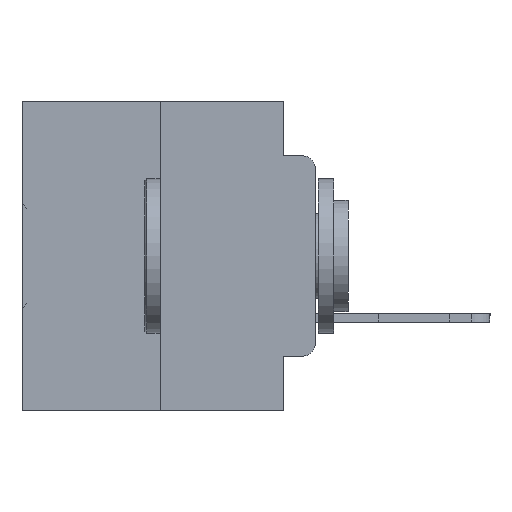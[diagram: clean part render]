
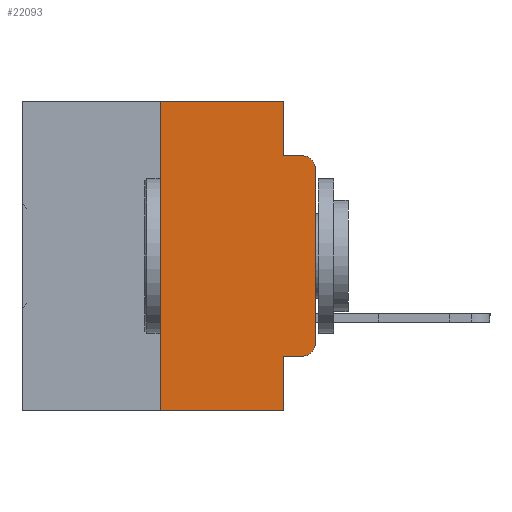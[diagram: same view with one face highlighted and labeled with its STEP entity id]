
A CAD part, left-side view. The second image highlights one B-rep face of the part: STEP entity #22093.
In plain terms, the highlighted planar face has unit normal (-1, 0, 0).
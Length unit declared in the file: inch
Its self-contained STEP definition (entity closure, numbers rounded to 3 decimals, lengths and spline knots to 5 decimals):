
#574 = DIRECTION ( 'NONE',  ( 0., -1., 0. ) ) ;
#651 = ORIENTED_EDGE ( 'NONE', *, *, #31635, .T. ) ;
#1986 = VERTEX_POINT ( 'NONE', #10382 ) ;
#2299 = LINE ( 'NONE', #29504, #22813 ) ;
#2353 = EDGE_CURVE ( 'NONE', #3374, #7126, #15050, .T. ) ;
#3009 = LINE ( 'NONE', #32769, #9323 ) ;
#3374 = VERTEX_POINT ( 'NONE', #23707 ) ;
#3595 = ORIENTED_EDGE ( 'NONE', *, *, #14703, .F. ) ;
#3640 = VERTEX_POINT ( 'NONE', #32210 ) ;
#3827 = VECTOR ( 'NONE', #5466, 39.37008 ) ;
#4020 = CARTESIAN_POINT ( 'NONE',  ( 0., 0.051, -0.4115 ) ) ;
#4184 = VERTEX_POINT ( 'NONE', #4714 ) ;
#4243 = DIRECTION ( 'NONE',  ( 0., 0., 1. ) ) ;
#4461 = PLANE ( 'NONE',  #11109 ) ;
#4573 = CARTESIAN_POINT ( 'NONE',  ( 0., 0.25, 0. ) ) ;
#4714 = CARTESIAN_POINT ( 'NONE',  ( 0., 0.02, -0.4115 ) ) ;
#4832 = EDGE_LOOP ( 'NONE', ( #13636, #28658, #15307, #29481, #3595, #25750, #12390, #14065, #28260, #651 ) ) ;
#5072 = CIRCLE ( 'NONE', #5090, 0.02 ) ;
#5090 = AXIS2_PLACEMENT_3D ( 'NONE', #6745, #25409, #9458 ) ;
#5247 = AXIS2_PLACEMENT_3D ( 'NONE', #12207, #30842, #14886 ) ;
#5418 = CARTESIAN_POINT ( 'NONE',  ( 0., 0.051, -0.5 ) ) ;
#5466 = DIRECTION ( 'NONE',  ( 0., -1., 0. ) ) ;
#5937 = DIRECTION ( 'NONE',  ( 0., 0., -1. ) ) ;
#5942 = CARTESIAN_POINT ( 'NONE',  ( 0., 0.051, 0. ) ) ;
#6423 = EDGE_CURVE ( 'NONE', #7899, #7126, #32448, .T. ) ;
#6745 = CARTESIAN_POINT ( 'NONE',  ( 0., 0.02, -0.1085 ) ) ;
#7126 = VERTEX_POINT ( 'NONE', #5418 ) ;
#7775 = EDGE_CURVE ( 'NONE', #7899, #22373, #2299, .T. ) ;
#7899 = VERTEX_POINT ( 'NONE', #22678 ) ;
#7978 = VECTOR ( 'NONE', #5937, 39.37008 ) ;
#9323 = VECTOR ( 'NONE', #29981, 39.37008 ) ;
#9449 = DIRECTION ( 'NONE',  ( 0., -1., 0. ) ) ;
#9458 = DIRECTION ( 'NONE',  ( 0., 0., -1. ) ) ;
#9572 = EDGE_CURVE ( 'NONE', #3640, #28501, #3009, .T. ) ;
#9873 = DIRECTION ( 'NONE',  ( 0., 0., -1. ) ) ;
#10382 = CARTESIAN_POINT ( 'NONE',  ( 0., 0., -0.3915 ) ) ;
#11109 = AXIS2_PLACEMENT_3D ( 'NONE', #23176, #25838, #9873 ) ;
#11825 = CARTESIAN_POINT ( 'NONE',  ( 0., 0.051, -0.0885 ) ) ;
#12207 = CARTESIAN_POINT ( 'NONE',  ( 0., 0.02, -0.3915 ) ) ;
#12390 = ORIENTED_EDGE ( 'NONE', *, *, #6423, .T. ) ;
#13125 = EDGE_CURVE ( 'NONE', #28501, #32445, #19003, .T. ) ;
#13632 = CARTESIAN_POINT ( 'NONE',  ( 0., 0., -0.1085 ) ) ;
#13636 = ORIENTED_EDGE ( 'NONE', *, *, #16710, .T. ) ;
#14065 = ORIENTED_EDGE ( 'NONE', *, *, #2353, .F. ) ;
#14703 = EDGE_CURVE ( 'NONE', #22373, #3640, #24322, .T. ) ;
#14754 = VERTEX_POINT ( 'NONE', #13632 ) ;
#14863 = CIRCLE ( 'NONE', #5247, 0.02 ) ;
#14886 = DIRECTION ( 'NONE',  ( 0., 0., -1. ) ) ;
#14906 = EDGE_CURVE ( 'NONE', #14754, #32445, #5072, .T. ) ;
#15050 = LINE ( 'NONE', #5942, #7978 ) ;
#15307 = ORIENTED_EDGE ( 'NONE', *, *, #13125, .F. ) ;
#15806 = VECTOR ( 'NONE', #4243, 39.37008 ) ;
#16661 = LINE ( 'NONE', #28187, #15806 ) ;
#16710 = EDGE_CURVE ( 'NONE', #1986, #14754, #16661, .T. ) ;
#18183 = VECTOR ( 'NONE', #574, 39.37008 ) ;
#18245 = DIRECTION ( 'NONE',  ( 0., -1., 0. ) ) ;
#18366 = VECTOR ( 'NONE', #18245, 39.37008 ) ;
#19003 = LINE ( 'NONE', #19360, #18183 ) ;
#19360 = CARTESIAN_POINT ( 'NONE',  ( 0., 0.051, -0.0885 ) ) ;
#21495 = CARTESIAN_POINT ( 'NONE',  ( 0., 0.473, 0. ) ) ;
#22093 = ADVANCED_FACE ( 'NONE', ( #30084 ), #4461, .F. ) ;
#22373 = VERTEX_POINT ( 'NONE', #4573 ) ;
#22678 = CARTESIAN_POINT ( 'NONE',  ( 0., 0.25, -0.5 ) ) ;
#22813 = VECTOR ( 'NONE', #32181, 39.37008 ) ;
#23176 = CARTESIAN_POINT ( 'NONE',  ( 0., 0.473, 0. ) ) ;
#23707 = CARTESIAN_POINT ( 'NONE',  ( 0., 0.051, -0.4115 ) ) ;
#24322 = LINE ( 'NONE', #21495, #3827 ) ;
#25409 = DIRECTION ( 'NONE',  ( -1., 0., 0. ) ) ;
#25750 = ORIENTED_EDGE ( 'NONE', *, *, #7775, .F. ) ;
#25838 = DIRECTION ( 'NONE',  ( 1., 0., 0. ) ) ;
#26416 = LINE ( 'NONE', #4020, #33482 ) ;
#28187 = CARTESIAN_POINT ( 'NONE',  ( 0., 0., 0. ) ) ;
#28260 = ORIENTED_EDGE ( 'NONE', *, *, #33421, .T. ) ;
#28501 = VERTEX_POINT ( 'NONE', #11825 ) ;
#28658 = ORIENTED_EDGE ( 'NONE', *, *, #14906, .T. ) ;
#28787 = CARTESIAN_POINT ( 'NONE',  ( 0., 0.473, -0.5 ) ) ;
#29481 = ORIENTED_EDGE ( 'NONE', *, *, #9572, .F. ) ;
#29504 = CARTESIAN_POINT ( 'NONE',  ( 0., 0.25, 0. ) ) ;
#29981 = DIRECTION ( 'NONE',  ( 0., 0., -1. ) ) ;
#30084 = FACE_OUTER_BOUND ( 'NONE', #4832, .T. ) ;
#30842 = DIRECTION ( 'NONE',  ( -1., 0., 0. ) ) ;
#31635 = EDGE_CURVE ( 'NONE', #4184, #1986, #14863, .T. ) ;
#32181 = DIRECTION ( 'NONE',  ( 0., 0., 1. ) ) ;
#32210 = CARTESIAN_POINT ( 'NONE',  ( 0., 0.051, 0. ) ) ;
#32445 = VERTEX_POINT ( 'NONE', #34163 ) ;
#32448 = LINE ( 'NONE', #28787, #18366 ) ;
#32769 = CARTESIAN_POINT ( 'NONE',  ( 0., 0.051, 0. ) ) ;
#33421 = EDGE_CURVE ( 'NONE', #3374, #4184, #26416, .T. ) ;
#33482 = VECTOR ( 'NONE', #9449, 39.37008 ) ;
#34163 = CARTESIAN_POINT ( 'NONE',  ( 0., 0.02, -0.0885 ) ) ;
